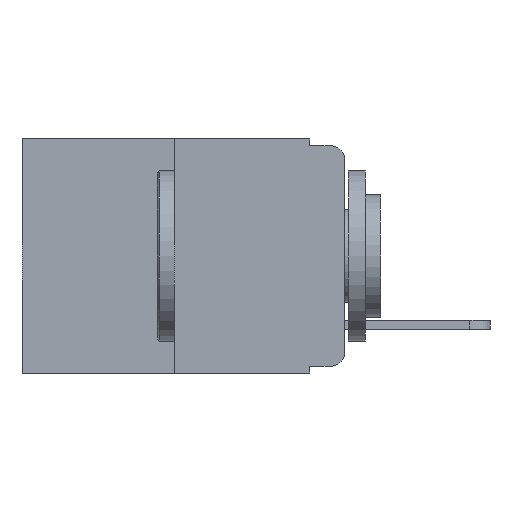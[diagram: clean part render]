
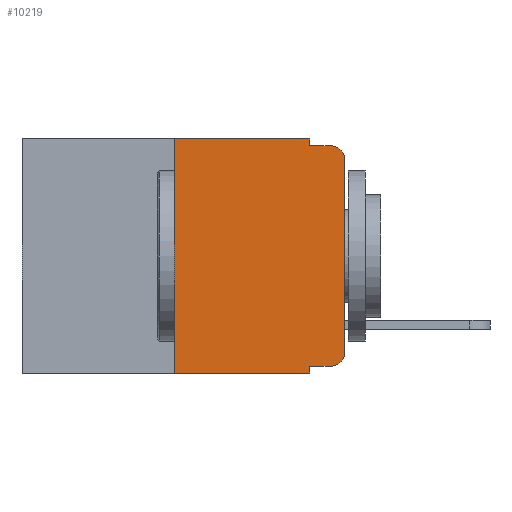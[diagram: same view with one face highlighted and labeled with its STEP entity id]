
A CAD part, left-side view. The second image highlights one B-rep face of the part: STEP entity #10219.
In plain terms, the highlighted planar face has unit normal (-1, 0, 0).
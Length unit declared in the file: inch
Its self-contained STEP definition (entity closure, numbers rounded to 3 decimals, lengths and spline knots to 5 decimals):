
#74 = LINE ( 'NONE', #6047, #5956 ) ;
#167 = VERTEX_POINT ( 'NONE', #12646 ) ;
#422 = DIRECTION ( 'NONE',  ( 0., -1., 0. ) ) ;
#437 = CARTESIAN_POINT ( 'NONE',  ( 0., 0.473, 0. ) ) ;
#502 = CIRCLE ( 'NONE', #12266, 0.02 ) ;
#939 = FACE_OUTER_BOUND ( 'NONE', #5648, .T. ) ;
#1099 = DIRECTION ( 'NONE',  ( 0., -1., 0. ) ) ;
#1179 = CARTESIAN_POINT ( 'NONE',  ( 0., 0.051, -0.333 ) ) ;
#1270 = CARTESIAN_POINT ( 'NONE',  ( 0., 0., 0. ) ) ;
#1292 = CARTESIAN_POINT ( 'NONE',  ( 0., 0.25, 0. ) ) ;
#1395 = CARTESIAN_POINT ( 'NONE',  ( 0., 0.473, -0.343 ) ) ;
#1429 = DIRECTION ( 'NONE',  ( 0., -1., 0. ) ) ;
#1672 = LINE ( 'NONE', #1964, #7395 ) ;
#1677 = CARTESIAN_POINT ( 'NONE',  ( 0., 0., -0.313 ) ) ;
#1964 = CARTESIAN_POINT ( 'NONE',  ( 0., 0.051, 0. ) ) ;
#2015 = CARTESIAN_POINT ( 'NONE',  ( 0., 0.051, -0.01 ) ) ;
#2621 = CARTESIAN_POINT ( 'NONE',  ( 0., 0.051, 0. ) ) ;
#3093 = EDGE_CURVE ( 'NONE', #3221, #7896, #10009, .T. ) ;
#3183 = VERTEX_POINT ( 'NONE', #11513 ) ;
#3221 = VERTEX_POINT ( 'NONE', #1292 ) ;
#3294 = DIRECTION ( 'NONE',  ( 0., 0., -1. ) ) ;
#3307 = DIRECTION ( 'NONE',  ( -1., 0., 0. ) ) ;
#3542 = DIRECTION ( 'NONE',  ( 0., -1., 0. ) ) ;
#3620 = AXIS2_PLACEMENT_3D ( 'NONE', #11312, #12577, #10433 ) ;
#4292 = ORIENTED_EDGE ( 'NONE', *, *, #11760, .T. ) ;
#4666 = ORIENTED_EDGE ( 'NONE', *, *, #10587, .F. ) ;
#4866 = VECTOR ( 'NONE', #422, 39.37008 ) ;
#4933 = VECTOR ( 'NONE', #1429, 39.37008 ) ;
#5148 = ORIENTED_EDGE ( 'NONE', *, *, #3093, .F. ) ;
#5496 = ORIENTED_EDGE ( 'NONE', *, *, #8485, .T. ) ;
#5585 = CARTESIAN_POINT ( 'NONE',  ( 0., 0.051, -0.01 ) ) ;
#5590 = LINE ( 'NONE', #1395, #4933 ) ;
#5648 = EDGE_LOOP ( 'NONE', ( #4292, #9984, #7042, #12200, #5148, #4666, #7382, #8651, #8006, #5496 ) ) ;
#5956 = VECTOR ( 'NONE', #10908, 39.37008 ) ;
#6047 = CARTESIAN_POINT ( 'NONE',  ( 0., 0.25, 0. ) ) ;
#6140 = DIRECTION ( 'NONE',  ( 0., 0., -1. ) ) ;
#6240 = CARTESIAN_POINT ( 'NONE',  ( 0., 0.25, -0.343 ) ) ;
#6600 = VECTOR ( 'NONE', #3542, 39.37008 ) ;
#6939 = VECTOR ( 'NONE', #1099, 39.37008 ) ;
#6998 = VERTEX_POINT ( 'NONE', #6240 ) ;
#7042 = ORIENTED_EDGE ( 'NONE', *, *, #11236, .F. ) ;
#7224 = VECTOR ( 'NONE', #13309, 39.37008 ) ;
#7348 = EDGE_CURVE ( 'NONE', #6998, #8400, #5590, .T. ) ;
#7382 = ORIENTED_EDGE ( 'NONE', *, *, #7348, .T. ) ;
#7395 = VECTOR ( 'NONE', #6140, 39.37008 ) ;
#7606 = CARTESIAN_POINT ( 'NONE',  ( 0., 0.02, -0.333 ) ) ;
#7851 = CIRCLE ( 'NONE', #9820, 0.02 ) ;
#7896 = VERTEX_POINT ( 'NONE', #2621 ) ;
#8006 = ORIENTED_EDGE ( 'NONE', *, *, #9495, .T. ) ;
#8400 = VERTEX_POINT ( 'NONE', #9679 ) ;
#8485 = EDGE_CURVE ( 'NONE', #11050, #11993, #502, .T. ) ;
#8548 = CARTESIAN_POINT ( 'NONE',  ( 0., 0.051, -0.333 ) ) ;
#8651 = ORIENTED_EDGE ( 'NONE', *, *, #10169, .F. ) ;
#8699 = DIRECTION ( 'NONE',  ( 0., 0., -1. ) ) ;
#8750 = DIRECTION ( 'NONE',  ( -1., 0., 0. ) ) ;
#8780 = CARTESIAN_POINT ( 'NONE',  ( 0., 0.02, -0.313 ) ) ;
#8834 = VECTOR ( 'NONE', #12471, 39.37008 ) ;
#8899 = VERTEX_POINT ( 'NONE', #5585 ) ;
#9151 = CARTESIAN_POINT ( 'NONE',  ( 0., 0.02, -0.03 ) ) ;
#9495 = EDGE_CURVE ( 'NONE', #10665, #11050, #9677, .T. ) ;
#9677 = LINE ( 'NONE', #1179, #6939 ) ;
#9679 = CARTESIAN_POINT ( 'NONE',  ( 0., 0.051, -0.343 ) ) ;
#9820 = AXIS2_PLACEMENT_3D ( 'NONE', #9151, #3307, #3294 ) ;
#9984 = ORIENTED_EDGE ( 'NONE', *, *, #11721, .T. ) ;
#10009 = LINE ( 'NONE', #437, #4866 ) ;
#10056 = CARTESIAN_POINT ( 'NONE',  ( 0., 0.051, 0. ) ) ;
#10169 = EDGE_CURVE ( 'NONE', #10665, #8400, #1672, .T. ) ;
#10219 = ADVANCED_FACE ( 'NONE', ( #939 ), #10228, .F. ) ;
#10228 = PLANE ( 'NONE',  #3620 ) ;
#10286 = LINE ( 'NONE', #1270, #7224 ) ;
#10433 = DIRECTION ( 'NONE',  ( 0., 0., -1. ) ) ;
#10587 = EDGE_CURVE ( 'NONE', #6998, #3221, #74, .T. ) ;
#10665 = VERTEX_POINT ( 'NONE', #8548 ) ;
#10765 = EDGE_CURVE ( 'NONE', #7896, #8899, #11460, .T. ) ;
#10908 = DIRECTION ( 'NONE',  ( 0., 0., 1. ) ) ;
#11050 = VERTEX_POINT ( 'NONE', #7606 ) ;
#11236 = EDGE_CURVE ( 'NONE', #8899, #167, #11890, .T. ) ;
#11312 = CARTESIAN_POINT ( 'NONE',  ( 0., 0.473, 0. ) ) ;
#11460 = LINE ( 'NONE', #10056, #8834 ) ;
#11513 = CARTESIAN_POINT ( 'NONE',  ( 0., 0., -0.03 ) ) ;
#11721 = EDGE_CURVE ( 'NONE', #3183, #167, #7851, .T. ) ;
#11760 = EDGE_CURVE ( 'NONE', #11993, #3183, #10286, .T. ) ;
#11890 = LINE ( 'NONE', #2015, #6600 ) ;
#11993 = VERTEX_POINT ( 'NONE', #1677 ) ;
#12200 = ORIENTED_EDGE ( 'NONE', *, *, #10765, .F. ) ;
#12266 = AXIS2_PLACEMENT_3D ( 'NONE', #8780, #8750, #8699 ) ;
#12471 = DIRECTION ( 'NONE',  ( 0., 0., -1. ) ) ;
#12577 = DIRECTION ( 'NONE',  ( 1., 0., 0. ) ) ;
#12646 = CARTESIAN_POINT ( 'NONE',  ( 0., 0.02, -0.01 ) ) ;
#13309 = DIRECTION ( 'NONE',  ( 0., 0., 1. ) ) ;
